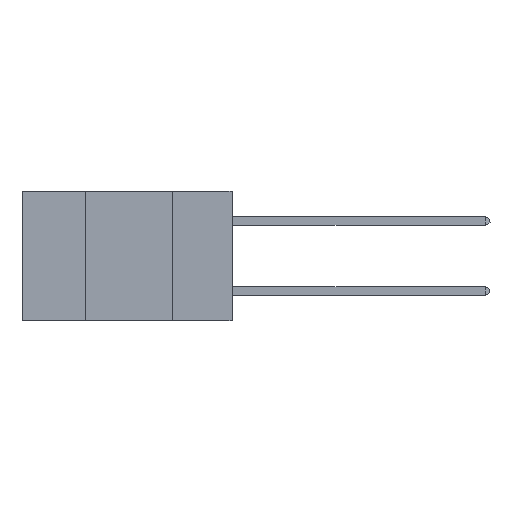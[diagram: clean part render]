
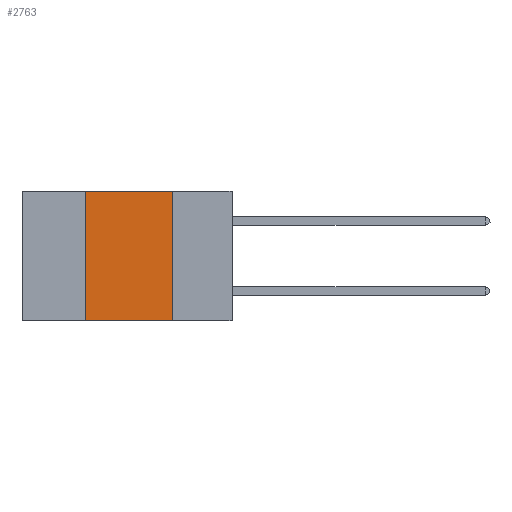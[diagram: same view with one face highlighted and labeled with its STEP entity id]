
A CAD part, left-side view. The second image highlights one B-rep face of the part: STEP entity #2763.
In plain terms, the highlighted planar face has unit normal (-1, 0, 0).
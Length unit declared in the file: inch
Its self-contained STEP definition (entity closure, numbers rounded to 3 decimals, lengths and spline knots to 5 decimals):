
#686 = LINE ( 'NONE', #10925, #15903 ) ;
#945 = ORIENTED_EDGE ( 'NONE', *, *, #7958, .T. ) ;
#2447 = ORIENTED_EDGE ( 'NONE', *, *, #16463, .F. ) ;
#2763 = ADVANCED_FACE ( 'NONE', ( #4724 ), #5838, .F. ) ;
#3361 = VECTOR ( 'NONE', #8043, 39.37008 ) ;
#4724 = FACE_OUTER_BOUND ( 'NONE', #8123, .T. ) ;
#4738 = VECTOR ( 'NONE', #18918, 39.37008 ) ;
#5046 = DIRECTION ( 'NONE',  ( 0., 0., 1. ) ) ;
#5657 = CARTESIAN_POINT ( 'NONE',  ( 0., 0.6, 0. ) ) ;
#5759 = VERTEX_POINT ( 'NONE', #8812 ) ;
#5838 = PLANE ( 'NONE',  #7829 ) ;
#5916 = EDGE_CURVE ( 'NONE', #5759, #14237, #17597, .T. ) ;
#6093 = DIRECTION ( 'NONE',  ( 0., 0., -1. ) ) ;
#7748 = ORIENTED_EDGE ( 'NONE', *, *, #5916, .F. ) ;
#7829 = AXIS2_PLACEMENT_3D ( 'NONE', #14885, #11753, #6093 ) ;
#7859 = ORIENTED_EDGE ( 'NONE', *, *, #16349, .F. ) ;
#7958 = EDGE_CURVE ( 'NONE', #5759, #15288, #686, .T. ) ;
#8043 = DIRECTION ( 'NONE',  ( 0., 0., -1. ) ) ;
#8123 = EDGE_LOOP ( 'NONE', ( #7859, #2447, #7748, #945 ) ) ;
#8812 = CARTESIAN_POINT ( 'NONE',  ( 0., 0.42, -0.37 ) ) ;
#8821 = VECTOR ( 'NONE', #5046, 39.37008 ) ;
#9708 = VERTEX_POINT ( 'NONE', #17006 ) ;
#10857 = CARTESIAN_POINT ( 'NONE',  ( 0., 0.42, 0. ) ) ;
#10925 = CARTESIAN_POINT ( 'NONE',  ( 0., 0.6, -0.37 ) ) ;
#11128 = CARTESIAN_POINT ( 'NONE',  ( 0., 0.17, 0. ) ) ;
#11753 = DIRECTION ( 'NONE',  ( 1., 0., 0. ) ) ;
#11881 = LINE ( 'NONE', #5657, #4738 ) ;
#12330 = LINE ( 'NONE', #11128, #3361 ) ;
#14237 = VERTEX_POINT ( 'NONE', #16867 ) ;
#14885 = CARTESIAN_POINT ( 'NONE',  ( 0., 0.6, 0. ) ) ;
#15288 = VERTEX_POINT ( 'NONE', #16910 ) ;
#15903 = VECTOR ( 'NONE', #16701, 39.37008 ) ;
#16349 = EDGE_CURVE ( 'NONE', #9708, #15288, #12330, .T. ) ;
#16463 = EDGE_CURVE ( 'NONE', #14237, #9708, #11881, .T. ) ;
#16701 = DIRECTION ( 'NONE',  ( 0., -1., 0. ) ) ;
#16867 = CARTESIAN_POINT ( 'NONE',  ( 0., 0.42, 0. ) ) ;
#16910 = CARTESIAN_POINT ( 'NONE',  ( 0., 0.17, -0.37 ) ) ;
#17006 = CARTESIAN_POINT ( 'NONE',  ( 0., 0.17, 0. ) ) ;
#17597 = LINE ( 'NONE', #10857, #8821 ) ;
#18918 = DIRECTION ( 'NONE',  ( 0., -1., 0. ) ) ;
